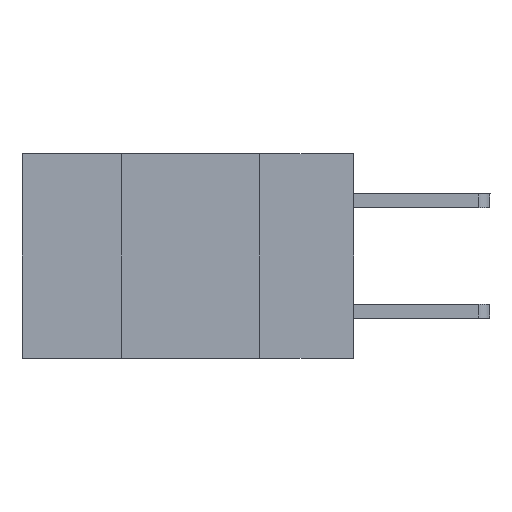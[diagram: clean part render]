
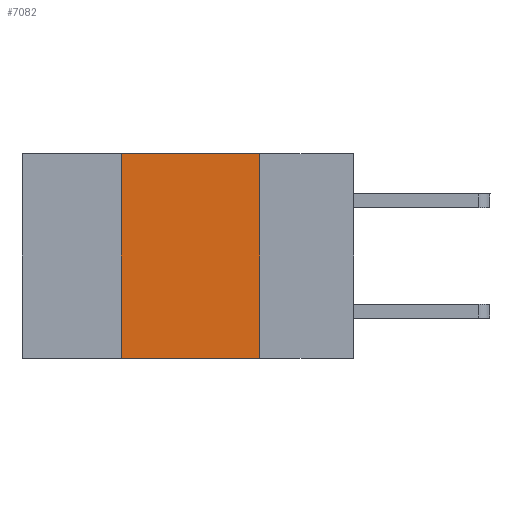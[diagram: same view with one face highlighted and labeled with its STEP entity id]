
A CAD part, left-side view. The second image highlights one B-rep face of the part: STEP entity #7082.
In plain terms, the highlighted planar face has unit normal (-1, 0, 0).
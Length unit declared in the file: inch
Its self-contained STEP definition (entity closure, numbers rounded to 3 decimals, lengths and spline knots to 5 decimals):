
#97 = DIRECTION ( 'NONE',  ( 0., 0., -1. ) ) ;
#694 = VECTOR ( 'NONE', #8470, 39.37008 ) ;
#1290 = VECTOR ( 'NONE', #5379, 39.37008 ) ;
#1313 = LINE ( 'NONE', #6813, #9248 ) ;
#1491 = CARTESIAN_POINT ( 'NONE',  ( 0., 0.42, -0.37 ) ) ;
#2575 = LINE ( 'NONE', #9432, #694 ) ;
#2825 = FACE_OUTER_BOUND ( 'NONE', #5626, .T. ) ;
#2858 = CARTESIAN_POINT ( 'NONE',  ( 0., 0.42, 0. ) ) ;
#2998 = ORIENTED_EDGE ( 'NONE', *, *, #6251, .F. ) ;
#3495 = ORIENTED_EDGE ( 'NONE', *, *, #8362, .F. ) ;
#4108 = VERTEX_POINT ( 'NONE', #2858 ) ;
#4319 = CARTESIAN_POINT ( 'NONE',  ( 0., 0.17, 0. ) ) ;
#4340 = ORIENTED_EDGE ( 'NONE', *, *, #4544, .F. ) ;
#4544 = EDGE_CURVE ( 'NONE', #10139, #4108, #2575, .T. ) ;
#4743 = EDGE_CURVE ( 'NONE', #10139, #12617, #1313, .T. ) ;
#4763 = CARTESIAN_POINT ( 'NONE',  ( 0., 0.17, -0.37 ) ) ;
#5168 = DIRECTION ( 'NONE',  ( 1., 0., 0. ) ) ;
#5379 = DIRECTION ( 'NONE',  ( 0., -1., 0. ) ) ;
#5626 = EDGE_LOOP ( 'NONE', ( #3495, #2998, #4340, #6201 ) ) ;
#6113 = CARTESIAN_POINT ( 'NONE',  ( 0., 0.6, 0. ) ) ;
#6201 = ORIENTED_EDGE ( 'NONE', *, *, #4743, .T. ) ;
#6251 = EDGE_CURVE ( 'NONE', #4108, #6302, #12202, .T. ) ;
#6302 = VERTEX_POINT ( 'NONE', #4319 ) ;
#6545 = DIRECTION ( 'NONE',  ( 0., 0., -1. ) ) ;
#6688 = VECTOR ( 'NONE', #6545, 39.37008 ) ;
#6813 = CARTESIAN_POINT ( 'NONE',  ( 0., 0.6, -0.37 ) ) ;
#7082 = ADVANCED_FACE ( 'NONE', ( #2825 ), #8008, .F. ) ;
#8008 = PLANE ( 'NONE',  #11152 ) ;
#8362 = EDGE_CURVE ( 'NONE', #6302, #12617, #12252, .T. ) ;
#8470 = DIRECTION ( 'NONE',  ( 0., 0., 1. ) ) ;
#9229 = CARTESIAN_POINT ( 'NONE',  ( 0., 0.6, 0. ) ) ;
#9248 = VECTOR ( 'NONE', #9815, 39.37008 ) ;
#9432 = CARTESIAN_POINT ( 'NONE',  ( 0., 0.42, 0. ) ) ;
#9815 = DIRECTION ( 'NONE',  ( 0., -1., 0. ) ) ;
#10139 = VERTEX_POINT ( 'NONE', #1491 ) ;
#11152 = AXIS2_PLACEMENT_3D ( 'NONE', #6113, #5168, #97 ) ;
#12202 = LINE ( 'NONE', #9229, #1290 ) ;
#12252 = LINE ( 'NONE', #12887, #6688 ) ;
#12617 = VERTEX_POINT ( 'NONE', #4763 ) ;
#12887 = CARTESIAN_POINT ( 'NONE',  ( 0., 0.17, 0. ) ) ;
